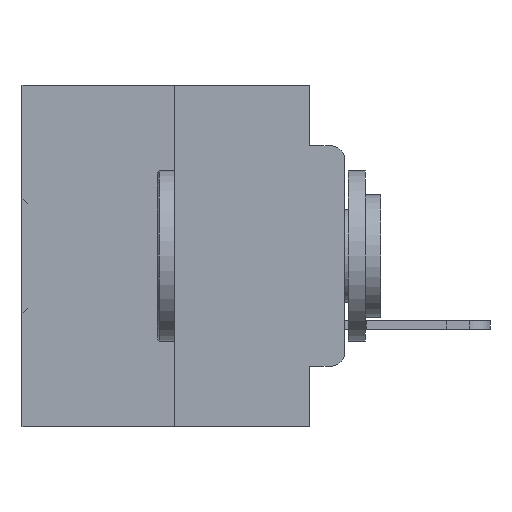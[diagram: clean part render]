
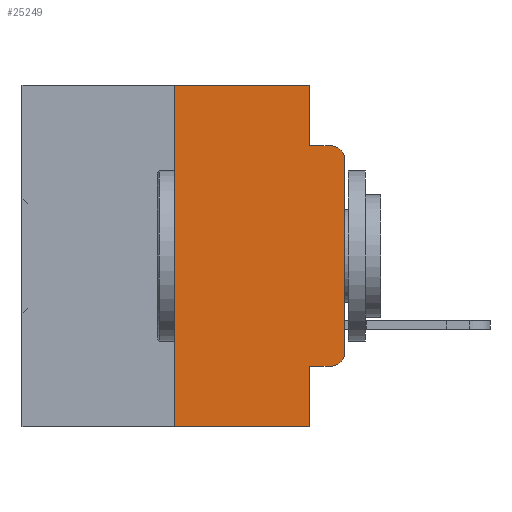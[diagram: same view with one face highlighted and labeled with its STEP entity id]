
A CAD part, left-side view. The second image highlights one B-rep face of the part: STEP entity #25249.
In plain terms, the highlighted planar face has unit normal (-1, 0, 0).
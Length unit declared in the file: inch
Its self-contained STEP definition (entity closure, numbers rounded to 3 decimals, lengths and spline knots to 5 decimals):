
#264 = CARTESIAN_POINT ( 'NONE',  ( 0., 0.051, 0. ) ) ;
#366 = VERTEX_POINT ( 'NONE', #2427 ) ;
#1399 = CARTESIAN_POINT ( 'NONE',  ( 0., 0.25, 0. ) ) ;
#1792 = EDGE_CURVE ( 'NONE', #10550, #20379, #29748, .T. ) ;
#1988 = ORIENTED_EDGE ( 'NONE', *, *, #31743, .T. ) ;
#2202 = LINE ( 'NONE', #5516, #9793 ) ;
#2373 = VECTOR ( 'NONE', #22752, 39.37008 ) ;
#2427 = CARTESIAN_POINT ( 'NONE',  ( 0., 0., -0.3915 ) ) ;
#2429 = AXIS2_PLACEMENT_3D ( 'NONE', #30172, #30127, #29964 ) ;
#3397 = ORIENTED_EDGE ( 'NONE', *, *, #11504, .T. ) ;
#3501 = VERTEX_POINT ( 'NONE', #9563 ) ;
#3599 = CIRCLE ( 'NONE', #19280, 0.02 ) ;
#3865 = EDGE_CURVE ( 'NONE', #22713, #24684, #15380, .T. ) ;
#4121 = ORIENTED_EDGE ( 'NONE', *, *, #21765, .T. ) ;
#4292 = DIRECTION ( 'NONE',  ( 0., 0., -1. ) ) ;
#4338 = DIRECTION ( 'NONE',  ( -1., 0., 0. ) ) ;
#4397 = CARTESIAN_POINT ( 'NONE',  ( 0., 0.02, -0.3915 ) ) ;
#5036 = LINE ( 'NONE', #12487, #13506 ) ;
#5507 = DIRECTION ( 'NONE',  ( 0., 0., 1. ) ) ;
#5516 = CARTESIAN_POINT ( 'NONE',  ( 0., 0.25, 0. ) ) ;
#5882 = ORIENTED_EDGE ( 'NONE', *, *, #22199, .T. ) ;
#6308 = ORIENTED_EDGE ( 'NONE', *, *, #14743, .T. ) ;
#8389 = EDGE_CURVE ( 'NONE', #3501, #16377, #32733, .T. ) ;
#8875 = DIRECTION ( 'NONE',  ( 0., 0., -1. ) ) ;
#9294 = DIRECTION ( 'NONE',  ( 0., -1., 0. ) ) ;
#9351 = ORIENTED_EDGE ( 'NONE', *, *, #3865, .F. ) ;
#9473 = VECTOR ( 'NONE', #8875, 39.37008 ) ;
#9502 = LINE ( 'NONE', #26705, #35036 ) ;
#9563 = CARTESIAN_POINT ( 'NONE',  ( 0., 0.051, -0.4115 ) ) ;
#9793 = VECTOR ( 'NONE', #5507, 39.37008 ) ;
#9907 = ORIENTED_EDGE ( 'NONE', *, *, #23390, .F. ) ;
#10155 = CARTESIAN_POINT ( 'NONE',  ( 0., 0., -0.1085 ) ) ;
#10312 = EDGE_CURVE ( 'NONE', #26666, #10550, #2202, .T. ) ;
#10550 = VERTEX_POINT ( 'NONE', #1399 ) ;
#10723 = PLANE ( 'NONE',  #13084 ) ;
#11504 = EDGE_CURVE ( 'NONE', #28733, #24684, #17073, .T. ) ;
#11632 = CARTESIAN_POINT ( 'NONE',  ( 0., 0.02, -0.0885 ) ) ;
#11847 = CARTESIAN_POINT ( 'NONE',  ( 0., 0.051, 0. ) ) ;
#12066 = ORIENTED_EDGE ( 'NONE', *, *, #1792, .F. ) ;
#12280 = ORIENTED_EDGE ( 'NONE', *, *, #10312, .F. ) ;
#12487 = CARTESIAN_POINT ( 'NONE',  ( 0., 0., 0. ) ) ;
#13084 = AXIS2_PLACEMENT_3D ( 'NONE', #30002, #35130, #19128 ) ;
#13401 = EDGE_LOOP ( 'NONE', ( #1988, #3397, #9351, #9907, #12066, #12280, #4121, #20418, #5882, #6308 ) ) ;
#13506 = VECTOR ( 'NONE', #31637, 39.37008 ) ;
#14029 = CARTESIAN_POINT ( 'NONE',  ( 0., 0.473, -0.5 ) ) ;
#14637 = CARTESIAN_POINT ( 'NONE',  ( 0., 0.02, -0.4115 ) ) ;
#14743 = EDGE_CURVE ( 'NONE', #31586, #366, #3599, .T. ) ;
#15380 = LINE ( 'NONE', #20249, #30008 ) ;
#15990 = VECTOR ( 'NONE', #9294, 39.37008 ) ;
#16377 = VERTEX_POINT ( 'NONE', #16711 ) ;
#16711 = CARTESIAN_POINT ( 'NONE',  ( 0., 0.051, -0.5 ) ) ;
#17073 = CIRCLE ( 'NONE', #2429, 0.02 ) ;
#19128 = DIRECTION ( 'NONE',  ( 0., 0., -1. ) ) ;
#19280 = AXIS2_PLACEMENT_3D ( 'NONE', #4397, #4338, #4292 ) ;
#20247 = DIRECTION ( 'NONE',  ( 0., -1., 0. ) ) ;
#20249 = CARTESIAN_POINT ( 'NONE',  ( 0., 0.051, -0.0885 ) ) ;
#20379 = VERTEX_POINT ( 'NONE', #11847 ) ;
#20418 = ORIENTED_EDGE ( 'NONE', *, *, #8389, .F. ) ;
#20421 = FACE_OUTER_BOUND ( 'NONE', #13401, .T. ) ;
#20929 = VECTOR ( 'NONE', #25092, 39.37008 ) ;
#21765 = EDGE_CURVE ( 'NONE', #26666, #16377, #35069, .T. ) ;
#22199 = EDGE_CURVE ( 'NONE', #3501, #31586, #9502, .T. ) ;
#22713 = VERTEX_POINT ( 'NONE', #28514 ) ;
#22752 = DIRECTION ( 'NONE',  ( 0., 0., -1. ) ) ;
#22911 = CARTESIAN_POINT ( 'NONE',  ( 0., 0.051, 0. ) ) ;
#23390 = EDGE_CURVE ( 'NONE', #20379, #22713, #24334, .T. ) ;
#24334 = LINE ( 'NONE', #264, #9473 ) ;
#24684 = VERTEX_POINT ( 'NONE', #11632 ) ;
#25092 = DIRECTION ( 'NONE',  ( 0., -1., 0. ) ) ;
#25249 = ADVANCED_FACE ( 'NONE', ( #20421 ), #10723, .F. ) ;
#26666 = VERTEX_POINT ( 'NONE', #29293 ) ;
#26705 = CARTESIAN_POINT ( 'NONE',  ( 0., 0.051, -0.4115 ) ) ;
#28514 = CARTESIAN_POINT ( 'NONE',  ( 0., 0.051, -0.0885 ) ) ;
#28733 = VERTEX_POINT ( 'NONE', #10155 ) ;
#29293 = CARTESIAN_POINT ( 'NONE',  ( 0., 0.25, -0.5 ) ) ;
#29379 = DIRECTION ( 'NONE',  ( 0., -1., 0. ) ) ;
#29748 = LINE ( 'NONE', #34562, #15990 ) ;
#29964 = DIRECTION ( 'NONE',  ( 0., 0., -1. ) ) ;
#30002 = CARTESIAN_POINT ( 'NONE',  ( 0., 0.473, 0. ) ) ;
#30008 = VECTOR ( 'NONE', #20247, 39.37008 ) ;
#30127 = DIRECTION ( 'NONE',  ( -1., 0., 0. ) ) ;
#30172 = CARTESIAN_POINT ( 'NONE',  ( 0., 0.02, -0.1085 ) ) ;
#31586 = VERTEX_POINT ( 'NONE', #14637 ) ;
#31637 = DIRECTION ( 'NONE',  ( 0., 0., 1. ) ) ;
#31743 = EDGE_CURVE ( 'NONE', #366, #28733, #5036, .T. ) ;
#32733 = LINE ( 'NONE', #22911, #2373 ) ;
#34562 = CARTESIAN_POINT ( 'NONE',  ( 0., 0.473, 0. ) ) ;
#35036 = VECTOR ( 'NONE', #29379, 39.37008 ) ;
#35069 = LINE ( 'NONE', #14029, #20929 ) ;
#35130 = DIRECTION ( 'NONE',  ( 1., 0., 0. ) ) ;
